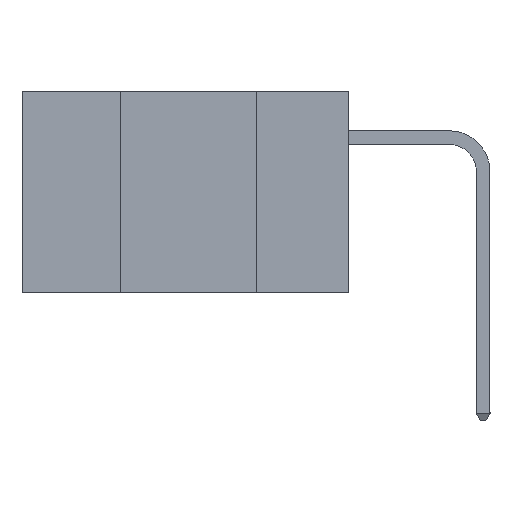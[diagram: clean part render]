
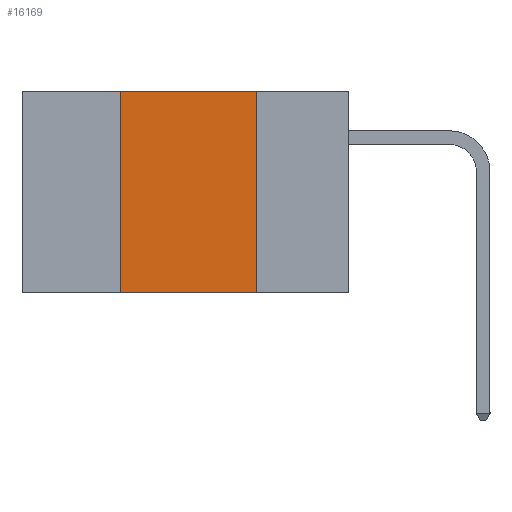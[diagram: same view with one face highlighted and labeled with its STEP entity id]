
A CAD part, left-side view. The second image highlights one B-rep face of the part: STEP entity #16169.
In plain terms, the highlighted planar face has unit normal (-1, 0, 0).
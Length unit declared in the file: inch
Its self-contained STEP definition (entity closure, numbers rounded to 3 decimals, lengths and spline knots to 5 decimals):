
#808 = PLANE ( 'NONE',  #16722 ) ;
#2257 = CARTESIAN_POINT ( 'NONE',  ( 0., 0.42, 0. ) ) ;
#2843 = VERTEX_POINT ( 'NONE', #8283 ) ;
#3233 = LINE ( 'NONE', #12258, #4235 ) ;
#4035 = ORIENTED_EDGE ( 'NONE', *, *, #25874, .F. ) ;
#4235 = VECTOR ( 'NONE', #5867, 39.37008 ) ;
#4680 = CARTESIAN_POINT ( 'NONE',  ( 0., 0.6, 0. ) ) ;
#5867 = DIRECTION ( 'NONE',  ( 0., 0., -1. ) ) ;
#6127 = CARTESIAN_POINT ( 'NONE',  ( 0., 0.17, 0. ) ) ;
#6316 = CARTESIAN_POINT ( 'NONE',  ( 0., 0.17, -0.37 ) ) ;
#6902 = ORIENTED_EDGE ( 'NONE', *, *, #10978, .T. ) ;
#7167 = DIRECTION ( 'NONE',  ( 0., 0., -1. ) ) ;
#8283 = CARTESIAN_POINT ( 'NONE',  ( 0., 0.42, -0.37 ) ) ;
#8501 = ORIENTED_EDGE ( 'NONE', *, *, #16683, .F. ) ;
#10322 = LINE ( 'NONE', #4680, #28154 ) ;
#10978 = EDGE_CURVE ( 'NONE', #2843, #21302, #36630, .T. ) ;
#11089 = VECTOR ( 'NONE', #16562, 39.37008 ) ;
#11430 = EDGE_LOOP ( 'NONE', ( #4035, #8501, #20475, #6902 ) ) ;
#12258 = CARTESIAN_POINT ( 'NONE',  ( 0., 0.17, 0. ) ) ;
#15650 = DIRECTION ( 'NONE',  ( 1., 0., 0. ) ) ;
#16169 = ADVANCED_FACE ( 'NONE', ( #26940 ), #808, .F. ) ;
#16562 = DIRECTION ( 'NONE',  ( 0., 0., 1. ) ) ;
#16683 = EDGE_CURVE ( 'NONE', #18364, #23770, #10322, .T. ) ;
#16722 = AXIS2_PLACEMENT_3D ( 'NONE', #29766, #15650, #7167 ) ;
#18364 = VERTEX_POINT ( 'NONE', #30236 ) ;
#20475 = ORIENTED_EDGE ( 'NONE', *, *, #29842, .F. ) ;
#21302 = VERTEX_POINT ( 'NONE', #6316 ) ;
#22022 = LINE ( 'NONE', #2257, #11089 ) ;
#23770 = VERTEX_POINT ( 'NONE', #6127 ) ;
#25874 = EDGE_CURVE ( 'NONE', #23770, #21302, #3233, .T. ) ;
#26940 = FACE_OUTER_BOUND ( 'NONE', #11430, .T. ) ;
#28154 = VECTOR ( 'NONE', #35747, 39.37008 ) ;
#29766 = CARTESIAN_POINT ( 'NONE',  ( 0., 0.6, 0. ) ) ;
#29842 = EDGE_CURVE ( 'NONE', #2843, #18364, #22022, .T. ) ;
#30236 = CARTESIAN_POINT ( 'NONE',  ( 0., 0.42, 0. ) ) ;
#30354 = VECTOR ( 'NONE', #30599, 39.37008 ) ;
#30599 = DIRECTION ( 'NONE',  ( 0., -1., 0. ) ) ;
#30785 = CARTESIAN_POINT ( 'NONE',  ( 0., 0.6, -0.37 ) ) ;
#35747 = DIRECTION ( 'NONE',  ( 0., -1., 0. ) ) ;
#36630 = LINE ( 'NONE', #30785, #30354 ) ;
